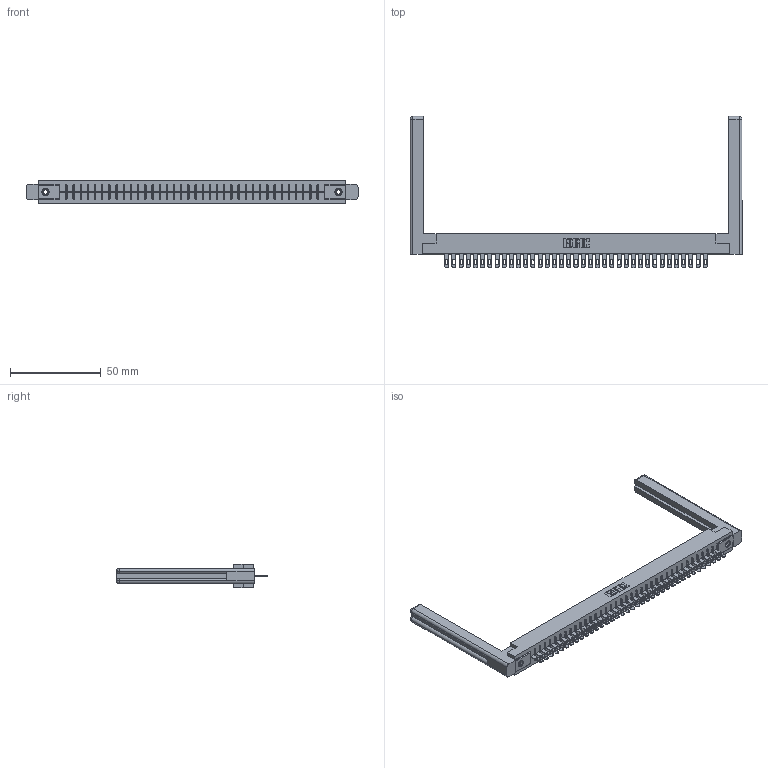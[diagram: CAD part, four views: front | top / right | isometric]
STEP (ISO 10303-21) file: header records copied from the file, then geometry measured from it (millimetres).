
FILE_DESCRIPTION (( 'STEP AP203' ), '1' );
FILE_NAME ('316-037-500-158.STEP', '2018-07-31T04:38:30', ( '' ), ( '' ), 'SwSTEP 2.0', 'SolidWorks 2016', '' );
FILE_SCHEMA (( 'CONFIG_CONTROL_DESIGN' ));
Length unit declared in the file: inch
Products named in the file (5): 306 Part_.156 Dia; 306-290-001_100; 345-250-001_345-250-001-102; 307-220-058; 316-037-500-158
Assembly tree (42 placements, depth 2):
  316-037-500-158
    306 Part_.156 Dia
    306-290-001_100  x37
    345-250-001_345-250-001-102  x2
    307-220-058  x2
Bounding box: 183.24 x 83.52 x 12.7 mm (x, y, z)
Volume: 27415.7 mm3; surface area: 26590.6 mm2
Topology: 42 solids, 42 shells, 3070 faces, 8625 edges, 5538 vertices
Faces by surface type: plane 2002, cylinder 896, sphere 148, cone 12, torus 12
Entity records: 37949 total; most frequent: CARTESIAN_POINT 6381, ORIENTED_EDGE 6268, DIRECTION 6248, EDGE_CURVE 3134, LINE 2442, VECTOR 2442, VERTEX_POINT 1982, AXIS2_PLACEMENT_3D 1903
